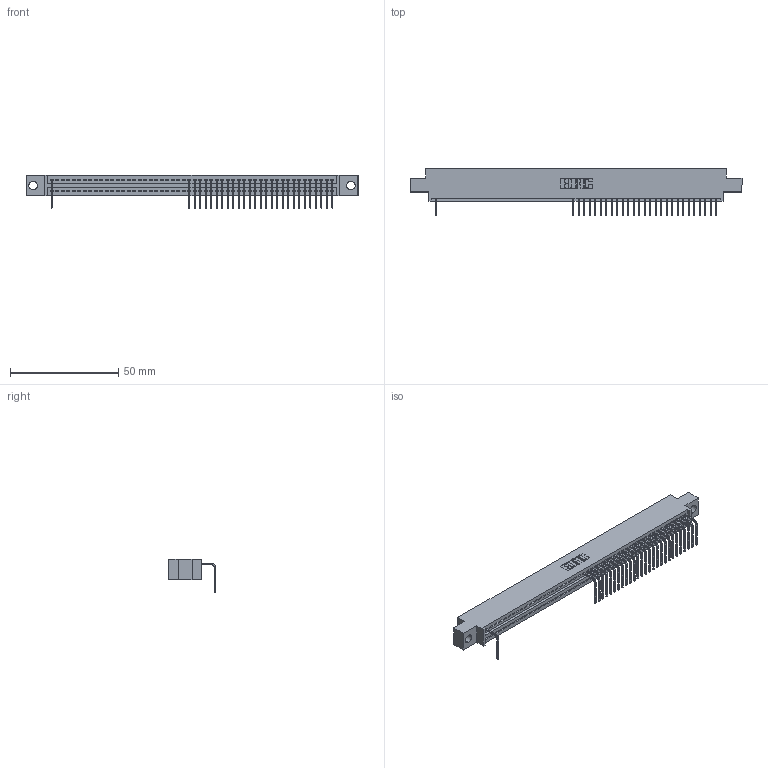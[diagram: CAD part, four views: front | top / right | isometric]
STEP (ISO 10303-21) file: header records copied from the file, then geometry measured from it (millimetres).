
FILE_DESCRIPTION (( 'STEP AP203' ), '1' );
FILE_NAME ('345-052-558-604.STEP', '2018-09-23T00:29:44', ( '' ), ( '' ), 'SwSTEP 2.0', 'SolidWorks 2016', '' );
FILE_SCHEMA (( 'CONFIG_CONTROL_DESIGN' ));
Length unit declared in the file: inch
Products named in the file (3): 345-292-001_558 Tail - 2; 345-052-558-604; 345 Part_0.170 Offset - 0.156 Dia-TH
Assembly tree (29 placements, depth 2):
  345-052-558-604
    345 Part_0.170 Offset - 0.156 Dia-TH
    345-292-001_558 Tail - 2  x28
Bounding box: 153.29 x 21.83 x 15.37 mm (x, y, z)
Volume: 14258.7 mm3; surface area: 18108.5 mm2
Topology: 29 solids, 29 shells, 2194 faces, 6745 edges, 4458 vertices
Faces by surface type: plane 1596, cylinder 598
Entity records: 37241 total; most frequent: ORIENTED_EDGE 6578, CARTESIAN_POINT 6568, DIRECTION 5693, EDGE_CURVE 3289, VECTOR 2949, LINE 2949, VERTEX_POINT 2190, AXIS2_PLACEMENT_3D 1372
